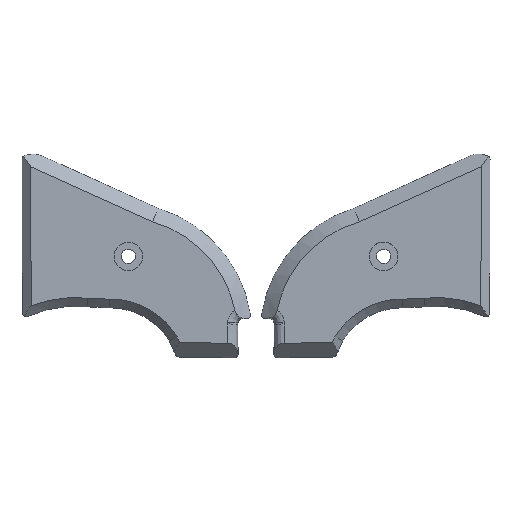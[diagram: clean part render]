
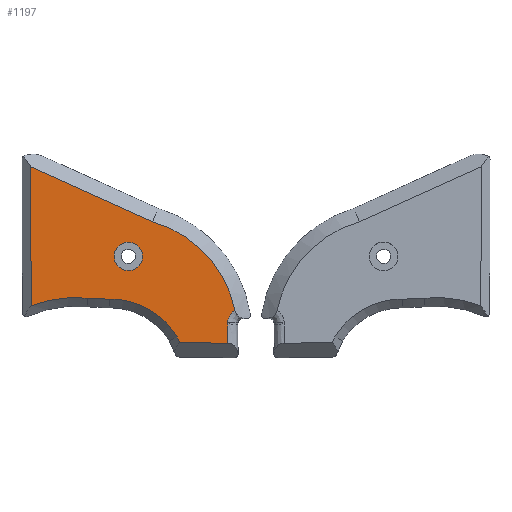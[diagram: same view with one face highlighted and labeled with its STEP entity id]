
A CAD part, top view. The second image highlights one B-rep face of the part: STEP entity #1197.
In plain terms, the highlighted planar face has unit normal (0, 0, 1).
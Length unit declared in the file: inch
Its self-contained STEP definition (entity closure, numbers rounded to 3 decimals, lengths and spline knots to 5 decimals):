
#38=B_SPLINE_CURVE_WITH_KNOTS('',3,(#1856,#1857,#1858,#1859),
 .UNSPECIFIED.,.F.,.F.,(4,4),(-1.07364,-0.39578),
 .UNSPECIFIED.);
#39=B_SPLINE_CURVE_WITH_KNOTS('',3,(#1861,#1862,#1863,#1864),
 .UNSPECIFIED.,.F.,.F.,(4,4),(-0.04305,0.00553),
 .UNSPECIFIED.);
#40=B_SPLINE_CURVE_WITH_KNOTS('',3,(#1866,#1867,#1868,#1869,#1870),
 .UNSPECIFIED.,.F.,.F.,(4,1,4),(-0.56305,-0.47097,-0.04305),
 .UNSPECIFIED.);
#79=LINE('',#1844,#163);
#80=LINE('',#1852,#164);
#81=LINE('',#1854,#165);
#82=LINE('',#1873,#166);
#163=VECTOR('',#1484,0.3937);
#164=VECTOR('',#1491,0.3937);
#165=VECTOR('',#1492,0.3937);
#166=VECTOR('',#1495,0.3937);
#276=FACE_BOUND('',#365,.T.);
#289=FACE_OUTER_BOUND('',#364,.T.);
#364=EDGE_LOOP('',(#837,#838,#839,#840,#841,#842,#843,#844,#845,#846,#847));
#365=EDGE_LOOP('',(#848));
#450=CIRCLE('',#1301,0.19685);
#453=CIRCLE('',#1306,1.78527);
#454=CIRCLE('',#1307,3.16162);
#455=CIRCLE('',#1308,1.08448);
#456=CIRCLE('',#1309,1.6175);
#515=VERTEX_POINT('',#1833);
#518=VERTEX_POINT('',#1842);
#519=VERTEX_POINT('',#1843);
#520=VERTEX_POINT('',#1845);
#521=VERTEX_POINT('',#1847);
#522=VERTEX_POINT('',#1849);
#523=VERTEX_POINT('',#1851);
#524=VERTEX_POINT('',#1853);
#525=VERTEX_POINT('',#1855);
#526=VERTEX_POINT('',#1860);
#527=VERTEX_POINT('',#1865);
#528=VERTEX_POINT('',#1871);
#639=EDGE_CURVE('',#515,#515,#450,.T.);
#643=EDGE_CURVE('',#518,#519,#79,.T.);
#644=EDGE_CURVE('',#520,#518,#453,.T.);
#645=EDGE_CURVE('',#521,#520,#454,.T.);
#646=EDGE_CURVE('',#522,#521,#455,.T.);
#647=EDGE_CURVE('',#523,#522,#80,.T.);
#648=EDGE_CURVE('',#524,#523,#81,.T.);
#649=EDGE_CURVE('',#525,#524,#38,.T.);
#650=EDGE_CURVE('',#526,#525,#39,.T.);
#651=EDGE_CURVE('',#527,#526,#40,.T.);
#652=EDGE_CURVE('',#528,#527,#456,.T.);
#653=EDGE_CURVE('',#519,#528,#82,.T.);
#837=ORIENTED_EDGE('',*,*,#643,.F.);
#838=ORIENTED_EDGE('',*,*,#644,.F.);
#839=ORIENTED_EDGE('',*,*,#645,.F.);
#840=ORIENTED_EDGE('',*,*,#646,.F.);
#841=ORIENTED_EDGE('',*,*,#647,.F.);
#842=ORIENTED_EDGE('',*,*,#648,.F.);
#843=ORIENTED_EDGE('',*,*,#649,.F.);
#844=ORIENTED_EDGE('',*,*,#650,.F.);
#845=ORIENTED_EDGE('',*,*,#651,.F.);
#846=ORIENTED_EDGE('',*,*,#652,.F.);
#847=ORIENTED_EDGE('',*,*,#653,.F.);
#848=ORIENTED_EDGE('',*,*,#639,.T.);
#1163=PLANE('',#1305);
#1197=ADVANCED_FACE('',(#289,#276),#1163,.F.);
#1301=AXIS2_PLACEMENT_3D('',#1834,#1473,#1474);
#1305=AXIS2_PLACEMENT_3D('',#1841,#1482,#1483);
#1306=AXIS2_PLACEMENT_3D('',#1846,#1485,#1486);
#1307=AXIS2_PLACEMENT_3D('',#1848,#1487,#1488);
#1308=AXIS2_PLACEMENT_3D('',#1850,#1489,#1490);
#1309=AXIS2_PLACEMENT_3D('',#1872,#1493,#1494);
#1473=DIRECTION('center_axis',(0.,0.,-1.));
#1474=DIRECTION('ref_axis',(-1.,0.,0.));
#1482=DIRECTION('center_axis',(0.,0.,-1.));
#1483=DIRECTION('ref_axis',(0.026,1.,0.));
#1484=DIRECTION('',(-0.003,1.,0.));
#1485=DIRECTION('center_axis',(0.,0.,1.));
#1486=DIRECTION('ref_axis',(-0.249,0.968,0.));
#1487=DIRECTION('center_axis',(0.,0.,-1.));
#1488=DIRECTION('ref_axis',(0.004,-1.,0.));
#1489=DIRECTION('center_axis',(0.,0.,1.));
#1490=DIRECTION('ref_axis',(-0.004,1.,0.));
#1491=DIRECTION('',(-0.405,0.915,0.));
#1492=DIRECTION('',(-1.,0.014,0.));
#1493=DIRECTION('center_axis',(0.,0.,-1.));
#1494=DIRECTION('ref_axis',(0.283,0.959,0.));
#1495=DIRECTION('',(0.911,-0.412,0.));
#1833=CARTESIAN_POINT('',(1.26454,-2.10286,1.09696));
#1834=CARTESIAN_POINT('Origin',(1.06769,-2.10286,1.09696));
#1841=CARTESIAN_POINT('Origin',(1.16979,-2.10243,1.09696));
#1842=CARTESIAN_POINT('',(-0.2793,-2.7859,1.09696));
#1843=CARTESIAN_POINT('',(-0.28577,-0.85851,1.09696));
#1844=CARTESIAN_POINT('',(-0.28384,-1.43282,1.09696));
#1845=CARTESIAN_POINT('',(0.5092,-2.68092,1.09696));
#1846=CARTESIAN_POINT('Origin',(0.34466,-4.45858,1.09696));
#1847=CARTESIAN_POINT('',(0.81169,-2.69435,1.09696));
#1848=CARTESIAN_POINT('Origin',(0.80059,0.46725,1.09696));
#1849=CARTESIAN_POINT('',(1.74489,-3.21996,1.09696));
#1850=CARTESIAN_POINT('Origin',(0.8155,-3.77883,1.09696));
#1851=CARTESIAN_POINT('',(1.77907,-3.29722,1.09696));
#1852=CARTESIAN_POINT('',(1.49265,-2.6498,1.09696));
#1853=CARTESIAN_POINT('',(2.44581,-3.30657,1.09696));
#1854=CARTESIAN_POINT('',(1.46308,-3.29279,1.09696));
#1855=CARTESIAN_POINT('',(2.44459,-3.0397,1.09696));
#1856=CARTESIAN_POINT('Ctrl Pts',(2.44459,-3.0397,1.09696));
#1857=CARTESIAN_POINT('Ctrl Pts',(2.445,-3.12866,1.09696));
#1858=CARTESIAN_POINT('Ctrl Pts',(2.44541,-3.21762,1.09696));
#1859=CARTESIAN_POINT('Ctrl Pts',(2.44581,-3.30657,1.09696));
#1860=CARTESIAN_POINT('',(2.44509,-3.02059,1.09696));
#1861=CARTESIAN_POINT('Ctrl Pts',(2.44509,-3.02059,1.09696));
#1862=CARTESIAN_POINT('Ctrl Pts',(2.44492,-3.02696,1.09696));
#1863=CARTESIAN_POINT('Ctrl Pts',(2.44475,-3.03333,1.09696));
#1864=CARTESIAN_POINT('Ctrl Pts',(2.44459,-3.0397,1.09696));
#1865=CARTESIAN_POINT('',(2.5457,-2.85239,1.09696));
#1866=CARTESIAN_POINT('Ctrl Pts',(2.54568,-2.85236,1.09696));
#1867=CARTESIAN_POINT('Ctrl Pts',(2.53516,-2.85834,1.09696));
#1868=CARTESIAN_POINT('Ctrl Pts',(2.47886,-2.89746,1.09696));
#1869=CARTESIAN_POINT('Ctrl Pts',(2.44656,-2.96445,1.09696));
#1870=CARTESIAN_POINT('Ctrl Pts',(2.44509,-3.02059,1.09696));
#1871=CARTESIAN_POINT('',(1.4057,-1.62343,1.09696));
#1872=CARTESIAN_POINT('Origin',(0.96146,-3.17873,1.09696));
#1873=CARTESIAN_POINT('',(1.3912,-1.61687,1.09696));
